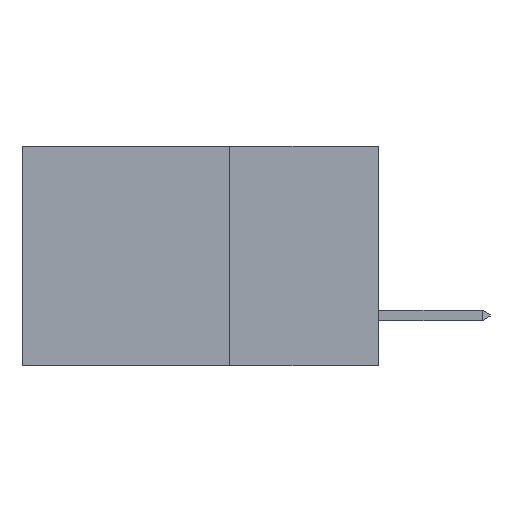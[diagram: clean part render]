
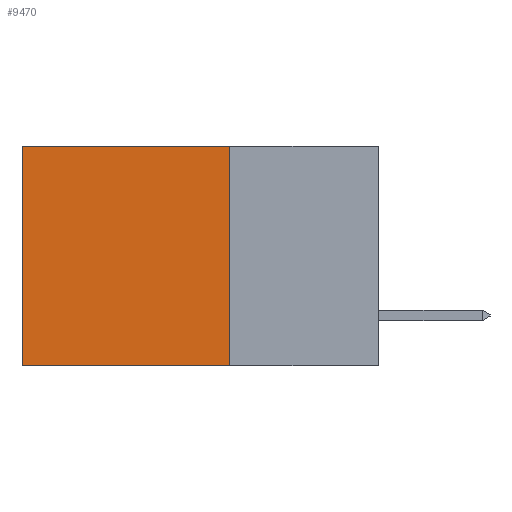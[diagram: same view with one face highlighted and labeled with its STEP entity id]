
A CAD part, left-side view. The second image highlights one B-rep face of the part: STEP entity #9470.
In plain terms, the highlighted planar face has unit normal (-1, 0, 0).
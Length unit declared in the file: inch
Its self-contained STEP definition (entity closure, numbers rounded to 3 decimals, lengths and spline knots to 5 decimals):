
#341 = EDGE_CURVE ( 'NONE', #3767, #16249, #9397, .T. ) ;
#346 = VECTOR ( 'NONE', #3087, 39.37008 ) ;
#2263 = CARTESIAN_POINT ( 'NONE',  ( 0.2615, 0.25, -0.37 ) ) ;
#2338 = EDGE_LOOP ( 'NONE', ( #10309, #2959, #21010, #4721 ) ) ;
#2959 = ORIENTED_EDGE ( 'NONE', *, *, #20276, .F. ) ;
#3087 = DIRECTION ( 'NONE',  ( 0., 1., 0. ) ) ;
#3320 = FACE_OUTER_BOUND ( 'NONE', #2338, .T. ) ;
#3626 = DIRECTION ( 'NONE',  ( 0., 0., -1. ) ) ;
#3767 = VERTEX_POINT ( 'NONE', #10709 ) ;
#4099 = VECTOR ( 'NONE', #14274, 39.37008 ) ;
#4284 = AXIS2_PLACEMENT_3D ( 'NONE', #16484, #15261, #15233 ) ;
#4638 = LINE ( 'NONE', #15995, #4099 ) ;
#4721 = ORIENTED_EDGE ( 'NONE', *, *, #16751, .T. ) ;
#8510 = LINE ( 'NONE', #15122, #21530 ) ;
#9397 = LINE ( 'NONE', #2263, #13931 ) ;
#9470 = ADVANCED_FACE ( 'NONE', ( #3320 ), #15459, .F. ) ;
#9552 = LINE ( 'NONE', #16911, #346 ) ;
#10304 = EDGE_CURVE ( 'NONE', #12414, #17537, #8510, .T. ) ;
#10309 = ORIENTED_EDGE ( 'NONE', *, *, #10304, .T. ) ;
#10709 = CARTESIAN_POINT ( 'NONE',  ( 0.2615, 0.25, 0. ) ) ;
#10952 = DIRECTION ( 'NONE',  ( 0., 0., -1. ) ) ;
#12414 = VERTEX_POINT ( 'NONE', #12962 ) ;
#12962 = CARTESIAN_POINT ( 'NONE',  ( 0.2615, 0.6, 0. ) ) ;
#13930 = CARTESIAN_POINT ( 'NONE',  ( 0.2615, 0.6, -0.37 ) ) ;
#13931 = VECTOR ( 'NONE', #3626, 39.37008 ) ;
#14274 = DIRECTION ( 'NONE',  ( 0., 1., 0. ) ) ;
#15122 = CARTESIAN_POINT ( 'NONE',  ( 0.2615, 0.6, -0.37 ) ) ;
#15233 = DIRECTION ( 'NONE',  ( 0., 0., -1. ) ) ;
#15261 = DIRECTION ( 'NONE',  ( 1., 0., 0. ) ) ;
#15459 = PLANE ( 'NONE',  #4284 ) ;
#15995 = CARTESIAN_POINT ( 'NONE',  ( 0.2615, 0.25, -0.37 ) ) ;
#16249 = VERTEX_POINT ( 'NONE', #18722 ) ;
#16484 = CARTESIAN_POINT ( 'NONE',  ( 0.2615, 0.25, -0.37 ) ) ;
#16751 = EDGE_CURVE ( 'NONE', #3767, #12414, #9552, .T. ) ;
#16911 = CARTESIAN_POINT ( 'NONE',  ( 0.2615, 0.25, 0. ) ) ;
#17537 = VERTEX_POINT ( 'NONE', #13930 ) ;
#18722 = CARTESIAN_POINT ( 'NONE',  ( 0.2615, 0.25, -0.37 ) ) ;
#20276 = EDGE_CURVE ( 'NONE', #16249, #17537, #4638, .T. ) ;
#21010 = ORIENTED_EDGE ( 'NONE', *, *, #341, .F. ) ;
#21530 = VECTOR ( 'NONE', #10952, 39.37008 ) ;
